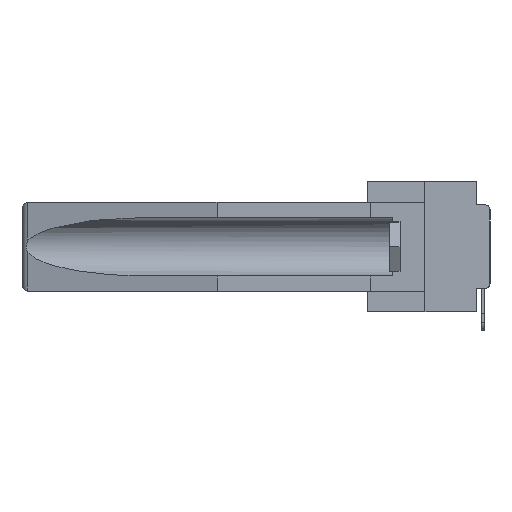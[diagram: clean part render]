
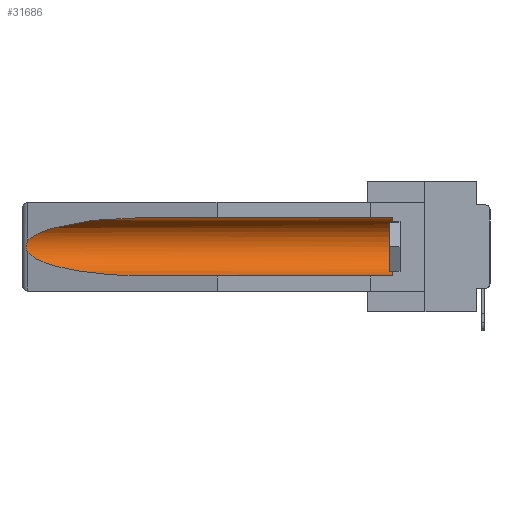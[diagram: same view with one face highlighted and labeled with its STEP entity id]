
A CAD part, left-side view. The second image highlights one B-rep face of the part: STEP entity #31686.
In plain terms, the highlighted cylindrical face has radius 2.857 mm (diameter 5.715 mm), a partial arc.
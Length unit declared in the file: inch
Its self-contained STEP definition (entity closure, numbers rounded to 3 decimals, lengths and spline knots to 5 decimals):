
#554 = CARTESIAN_POINT ( 'NONE',  ( 0.26654, 1.53092, -0.15636 ) ) ;
#2642 = CARTESIAN_POINT ( 'NONE',  ( 0.21114, 1.30732, -0.059 ) ) ;
#2814 = VERTEX_POINT ( 'NONE', #24619 ) ;
#3228 = CYLINDRICAL_SURFACE ( 'NONE', #29834, 0.1125 ) ;
#5603 = DIRECTION ( 'NONE',  ( 0., 1., 0. ) ) ;
#5639 = CARTESIAN_POINT ( 'NONE',  ( 0.26597, 1.52961, -0.15275 ) ) ;
#5989 = CARTESIAN_POINT ( 'NONE',  ( 0.2673, 1.53269, -0.17917 ) ) ;
#6749 = VERTEX_POINT ( 'NONE', #10591 ) ;
#6957 = CARTESIAN_POINT ( 'NONE',  ( 0.155, 1.07973, -0.284 ) ) ;
#6966 = LINE ( 'NONE', #8280, #14083 ) ;
#7615 = DIRECTION ( 'NONE',  ( 0., 0., 1. ) ) ;
#8087 = CARTESIAN_POINT ( 'NONE',  ( 0.26537, 1.52718, -0.19328 ) ) ;
#8280 = CARTESIAN_POINT ( 'NONE',  ( 0.155, -0.30754, -0.059 ) ) ;
#8807 = EDGE_CURVE ( 'NONE', #31425, #6749, #29670, .T. ) ;
#8998 = VERTEX_POINT ( 'NONE', #19105 ) ;
#9735 = DIRECTION ( 'NONE',  ( 0., -1., 0. ) ) ;
#9962 = FACE_OUTER_BOUND ( 'NONE', #29217, .T. ) ;
#10591 = CARTESIAN_POINT ( 'NONE',  ( 0.26537, 1.52718, -0.19328 ) ) ;
#11462 = VERTEX_POINT ( 'NONE', #31243 ) ;
#11745 = DIRECTION ( 'NONE',  ( 0., 0., 1. ) ) ;
#12715 = LINE ( 'NONE', #30627, #31344 ) ;
#13605 = ORIENTED_EDGE ( 'NONE', *, *, #29315, .T. ) ;
#13760 = VERTEX_POINT ( 'NONE', #23549 ) ;
#14083 = VECTOR ( 'NONE', #28657, 39.37008 ) ;
#14492 = DIRECTION ( 'NONE',  ( 0., 1., 0. ) ) ;
#15365 = CARTESIAN_POINT ( 'NONE',  ( 0.26537, 1.52718, -0.14972 ) ) ;
#15974 = AXIS2_PLACEMENT_3D ( 'NONE', #20251, #9735, #7615 ) ;
#16175 = CARTESIAN_POINT ( 'NONE',  ( 0.2675, 1.53308, -0.17534 ) ) ;
#16489 =( BOUNDED_CURVE ( )  B_SPLINE_CURVE ( 3, ( #30415, #2642, #27881, #15365 ),
 .UNSPECIFIED., .F., .F. ) 
 B_SPLINE_CURVE_WITH_KNOTS ( ( 4, 4 ),
 ( 4.71239, 6.08839 ),
 .UNSPECIFIED. ) 
 CURVE ( )  GEOMETRIC_REPRESENTATION_ITEM ( )  RATIONAL_B_SPLINE_CURVE ( ( 1., 0.848, 0.848, 1. ) ) 
 REPRESENTATION_ITEM ( '' )  );
#16953 = CIRCLE ( 'NONE', #15974, 0.1125 ) ;
#17356 = EDGE_CURVE ( 'NONE', #8998, #13760, #16953, .T. ) ;
#18271 = ORIENTED_EDGE ( 'NONE', *, *, #8807, .T. ) ;
#18740 = CARTESIAN_POINT ( 'NONE',  ( 0.26655, 1.53094, -0.18657 ) ) ;
#18827 = EDGE_CURVE ( 'NONE', #11462, #31425, #16489, .T. ) ;
#19105 = CARTESIAN_POINT ( 'NONE',  ( 0.155, 0.126, -0.284 ) ) ;
#20251 = CARTESIAN_POINT ( 'NONE',  ( 0.155, 0.126, -0.1715 ) ) ;
#22051 = CARTESIAN_POINT ( 'NONE',  ( 0.155, -0.30754, -0.1715 ) ) ;
#23248 = CARTESIAN_POINT ( 'NONE',  ( 0.2673, 1.5327, -0.16383 ) ) ;
#23549 = CARTESIAN_POINT ( 'NONE',  ( 0.155, 0.126, -0.059 ) ) ;
#23745 = ORIENTED_EDGE ( 'NONE', *, *, #17356, .T. ) ;
#23796 = ORIENTED_EDGE ( 'NONE', *, *, #27699, .T. ) ;
#24619 = CARTESIAN_POINT ( 'NONE',  ( 0.155, 1.07973, -0.284 ) ) ;
#25771 =( BOUNDED_CURVE ( )  B_SPLINE_CURVE ( 3, ( #27202, #27310, #32323, #6957 ),
 .UNSPECIFIED., .F., .F. ) 
 B_SPLINE_CURVE_WITH_KNOTS ( ( 4, 4 ),
 ( 0.1948, 1.5708 ),
 .UNSPECIFIED. ) 
 CURVE ( )  GEOMETRIC_REPRESENTATION_ITEM ( )  RATIONAL_B_SPLINE_CURVE ( ( 1., 0.848, 0.848, 1. ) ) 
 REPRESENTATION_ITEM ( '' )  );
#26349 = ORIENTED_EDGE ( 'NONE', *, *, #31959, .F. ) ;
#27202 = CARTESIAN_POINT ( 'NONE',  ( 0.26537, 1.52718, -0.19328 ) ) ;
#27310 = CARTESIAN_POINT ( 'NONE',  ( 0.25451, 1.48313, -0.24835 ) ) ;
#27699 = EDGE_CURVE ( 'NONE', #13760, #11462, #6966, .T. ) ;
#27881 = CARTESIAN_POINT ( 'NONE',  ( 0.25451, 1.48313, -0.09465 ) ) ;
#28457 = CARTESIAN_POINT ( 'NONE',  ( 0.2675, 1.53308, -0.16763 ) ) ;
#28657 = DIRECTION ( 'NONE',  ( 0., 1., 0. ) ) ;
#28691 = CARTESIAN_POINT ( 'NONE',  ( 0.26597, 1.5296, -0.19026 ) ) ;
#29217 = EDGE_LOOP ( 'NONE', ( #29346, #18271, #13605, #26349, #23745, #23796 ) ) ;
#29315 = EDGE_CURVE ( 'NONE', #6749, #2814, #25771, .T. ) ;
#29346 = ORIENTED_EDGE ( 'NONE', *, *, #18827, .T. ) ;
#29670 = B_SPLINE_CURVE_WITH_KNOTS ( 'NONE', 3,
 ( #31117, #5639, #554, #23248, #28457, #16175, #5989, #18740, #28691, #8087 ),
 .UNSPECIFIED., .F., .F.,
 ( 4, 2, 2, 2, 4 ),
 ( 0., 0.00029, 0.00058, 0.00087, 0.00117 ),
 .UNSPECIFIED. ) ;
#29834 = AXIS2_PLACEMENT_3D ( 'NONE', #22051, #14492, #11745 ) ;
#30415 = CARTESIAN_POINT ( 'NONE',  ( 0.155, 1.07973, -0.059 ) ) ;
#30627 = CARTESIAN_POINT ( 'NONE',  ( 0.155, -0.30754, -0.284 ) ) ;
#30885 = CARTESIAN_POINT ( 'NONE',  ( 0.26537, 1.52718, -0.14972 ) ) ;
#31117 = CARTESIAN_POINT ( 'NONE',  ( 0.26537, 1.52718, -0.14972 ) ) ;
#31243 = CARTESIAN_POINT ( 'NONE',  ( 0.155, 1.07973, -0.059 ) ) ;
#31344 = VECTOR ( 'NONE', #5603, 39.37008 ) ;
#31425 = VERTEX_POINT ( 'NONE', #30885 ) ;
#31686 = ADVANCED_FACE ( 'NONE', ( #9962 ), #3228, .F. ) ;
#31959 = EDGE_CURVE ( 'NONE', #8998, #2814, #12715, .T. ) ;
#32323 = CARTESIAN_POINT ( 'NONE',  ( 0.21114, 1.30732, -0.284 ) ) ;
